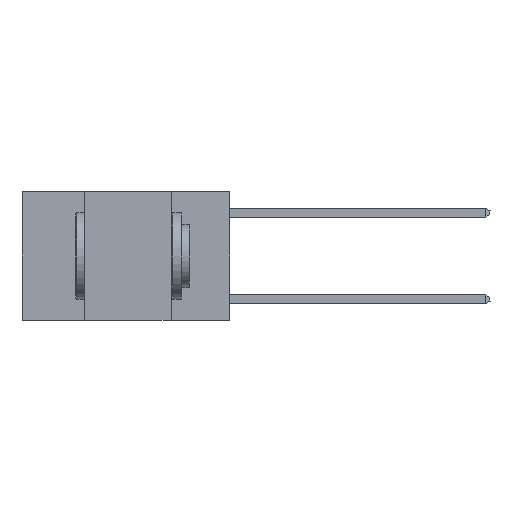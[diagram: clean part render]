
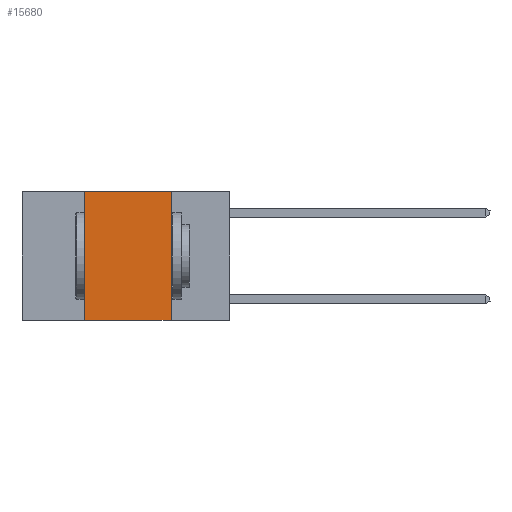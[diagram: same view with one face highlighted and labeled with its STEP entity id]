
A CAD part, left-side view. The second image highlights one B-rep face of the part: STEP entity #15680.
In plain terms, the highlighted planar face has unit normal (-1, 0, 0).
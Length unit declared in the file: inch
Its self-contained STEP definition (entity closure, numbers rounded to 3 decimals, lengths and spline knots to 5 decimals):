
#88 = CARTESIAN_POINT ( 'NONE',  ( 0., 0.42, 0. ) ) ;
#894 = VERTEX_POINT ( 'NONE', #6609 ) ;
#2122 = ORIENTED_EDGE ( 'NONE', *, *, #21646, .F. ) ;
#2275 = CARTESIAN_POINT ( 'NONE',  ( 0., 0.42, 0. ) ) ;
#2400 = DIRECTION ( 'NONE',  ( 0., 0., 1. ) ) ;
#3000 = EDGE_LOOP ( 'NONE', ( #18086, #19541, #2122, #20226 ) ) ;
#4349 = EDGE_CURVE ( 'NONE', #22481, #26236, #20010, .T. ) ;
#4820 = EDGE_CURVE ( 'NONE', #18967, #22481, #19695, .T. ) ;
#6498 = LINE ( 'NONE', #88, #17861 ) ;
#6609 = CARTESIAN_POINT ( 'NONE',  ( 0., 0.42, -0.37 ) ) ;
#7633 = VECTOR ( 'NONE', #29129, 39.37008 ) ;
#7749 = CARTESIAN_POINT ( 'NONE',  ( 0., 0.17, -0.37 ) ) ;
#9088 = AXIS2_PLACEMENT_3D ( 'NONE', #9092, #24879, #11378 ) ;
#9092 = CARTESIAN_POINT ( 'NONE',  ( 0., 0.6, 0. ) ) ;
#9602 = CARTESIAN_POINT ( 'NONE',  ( 0., 0.17, 0. ) ) ;
#9738 = VECTOR ( 'NONE', #13135, 39.37008 ) ;
#10544 = FACE_OUTER_BOUND ( 'NONE', #3000, .T. ) ;
#10889 = CARTESIAN_POINT ( 'NONE',  ( 0., 0.6, -0.37 ) ) ;
#11378 = DIRECTION ( 'NONE',  ( 0., 0., -1. ) ) ;
#13135 = DIRECTION ( 'NONE',  ( 0., -1., 0. ) ) ;
#15680 = ADVANCED_FACE ( 'NONE', ( #10544 ), #22614, .F. ) ;
#16185 = CARTESIAN_POINT ( 'NONE',  ( 0., 0.17, 0. ) ) ;
#17861 = VECTOR ( 'NONE', #2400, 39.37008 ) ;
#18086 = ORIENTED_EDGE ( 'NONE', *, *, #4349, .F. ) ;
#18967 = VERTEX_POINT ( 'NONE', #2275 ) ;
#19541 = ORIENTED_EDGE ( 'NONE', *, *, #4820, .F. ) ;
#19695 = LINE ( 'NONE', #26912, #7633 ) ;
#20010 = LINE ( 'NONE', #9602, #25322 ) ;
#20226 = ORIENTED_EDGE ( 'NONE', *, *, #22219, .T. ) ;
#21646 = EDGE_CURVE ( 'NONE', #894, #18967, #6498, .T. ) ;
#21729 = LINE ( 'NONE', #10889, #9738 ) ;
#22219 = EDGE_CURVE ( 'NONE', #894, #26236, #21729, .T. ) ;
#22481 = VERTEX_POINT ( 'NONE', #16185 ) ;
#22614 = PLANE ( 'NONE',  #9088 ) ;
#24879 = DIRECTION ( 'NONE',  ( 1., 0., 0. ) ) ;
#25322 = VECTOR ( 'NONE', #27624, 39.37008 ) ;
#26236 = VERTEX_POINT ( 'NONE', #7749 ) ;
#26912 = CARTESIAN_POINT ( 'NONE',  ( 0., 0.6, 0. ) ) ;
#27624 = DIRECTION ( 'NONE',  ( 0., 0., -1. ) ) ;
#29129 = DIRECTION ( 'NONE',  ( 0., -1., 0. ) ) ;
